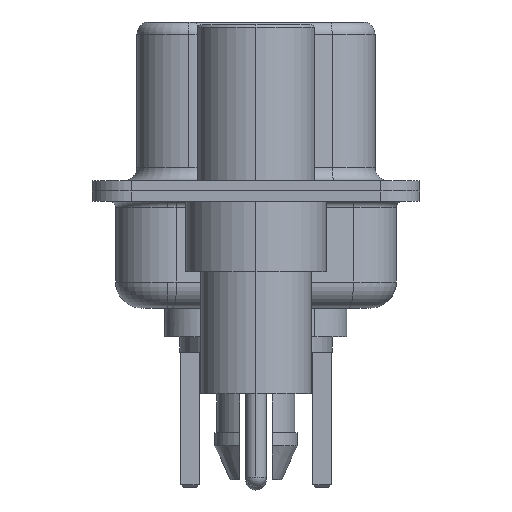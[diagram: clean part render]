
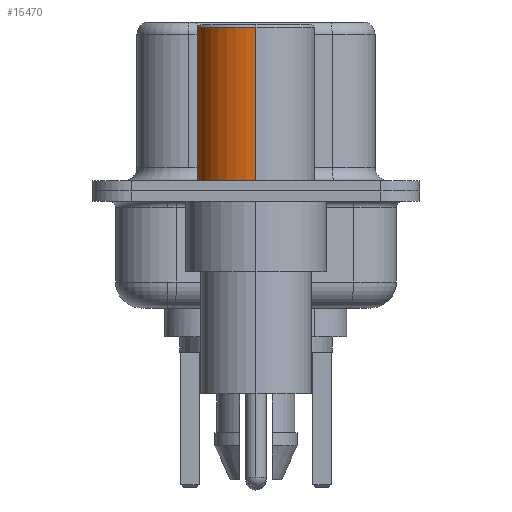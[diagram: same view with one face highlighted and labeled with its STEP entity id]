
A CAD part, left-side view. The second image highlights one B-rep face of the part: STEP entity #15470.
In plain terms, the highlighted cylindrical face has radius 2.25 mm (diameter 4.5 mm), a partial arc.
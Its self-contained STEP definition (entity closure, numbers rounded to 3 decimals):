
#314 = LINE ( 'NONE', #955, #7999 ) ;
#377 = CYLINDRICAL_SURFACE ( 'NONE', #14038, 2.25 ) ;
#939 = VERTEX_POINT ( 'NONE', #10428 ) ;
#955 = CARTESIAN_POINT ( 'NONE',  ( 2.25, 0., 0.581 ) ) ;
#1856 = ORIENTED_EDGE ( 'NONE', *, *, #6290, .F. ) ;
#2267 = DIRECTION ( 'NONE',  ( 0., 0., 1. ) ) ;
#2543 = CARTESIAN_POINT ( 'NONE',  ( -2.25, 0., 0.581 ) ) ;
#2818 = CARTESIAN_POINT ( 'NONE',  ( 0., 0., 6.3 ) ) ;
#4037 = AXIS2_PLACEMENT_3D ( 'NONE', #2818, #2267, #18164 ) ;
#4045 = DIRECTION ( 'NONE',  ( 0., 0., 1. ) ) ;
#5013 = DIRECTION ( 'NONE',  ( 0., 0., 1. ) ) ;
#5413 = VERTEX_POINT ( 'NONE', #14540 ) ;
#5988 = EDGE_LOOP ( 'NONE', ( #17477, #10867, #18941, #1856 ) ) ;
#6290 = EDGE_CURVE ( 'NONE', #6344, #939, #314, .T. ) ;
#6309 = EDGE_CURVE ( 'NONE', #939, #5413, #13166, .T. ) ;
#6344 = VERTEX_POINT ( 'NONE', #17605 ) ;
#7999 = VECTOR ( 'NONE', #10730, 1000. ) ;
#9061 = DIRECTION ( 'NONE',  ( 0., 0., 1. ) ) ;
#9410 = CARTESIAN_POINT ( 'NONE',  ( -2.25, 0., 0.4 ) ) ;
#10428 = CARTESIAN_POINT ( 'NONE',  ( 2.25, 0., 6.3 ) ) ;
#10730 = DIRECTION ( 'NONE',  ( 0., 0., 1. ) ) ;
#10867 = ORIENTED_EDGE ( 'NONE', *, *, #11239, .T. ) ;
#11218 = DIRECTION ( 'NONE',  ( 1., 0., 0. ) ) ;
#11239 = EDGE_CURVE ( 'NONE', #17035, #5413, #19163, .T. ) ;
#12386 = EDGE_CURVE ( 'NONE', #6344, #17035, #18930, .T. ) ;
#13166 = CIRCLE ( 'NONE', #4037, 2.25 ) ;
#14038 = AXIS2_PLACEMENT_3D ( 'NONE', #15828, #5013, #11218 ) ;
#14540 = CARTESIAN_POINT ( 'NONE',  ( -2.25, 0., 6.3 ) ) ;
#15470 = ADVANCED_FACE ( 'NONE', ( #16768 ), #377, .T. ) ;
#15621 = VECTOR ( 'NONE', #4045, 1000. ) ;
#15828 = CARTESIAN_POINT ( 'NONE',  ( 0., 0., 0.581 ) ) ;
#15897 = AXIS2_PLACEMENT_3D ( 'NONE', #18292, #9061, #19819 ) ;
#16768 = FACE_OUTER_BOUND ( 'NONE', #5988, .T. ) ;
#17035 = VERTEX_POINT ( 'NONE', #9410 ) ;
#17477 = ORIENTED_EDGE ( 'NONE', *, *, #12386, .T. ) ;
#17605 = CARTESIAN_POINT ( 'NONE',  ( 2.25, 0., 0.4 ) ) ;
#18164 = DIRECTION ( 'NONE',  ( 1., 0., 0. ) ) ;
#18292 = CARTESIAN_POINT ( 'NONE',  ( 0., 0., 0.4 ) ) ;
#18930 = CIRCLE ( 'NONE', #15897, 2.25 ) ;
#18941 = ORIENTED_EDGE ( 'NONE', *, *, #6309, .F. ) ;
#19163 = LINE ( 'NONE', #2543, #15621 ) ;
#19819 = DIRECTION ( 'NONE',  ( 1., 0., 0. ) ) ;
